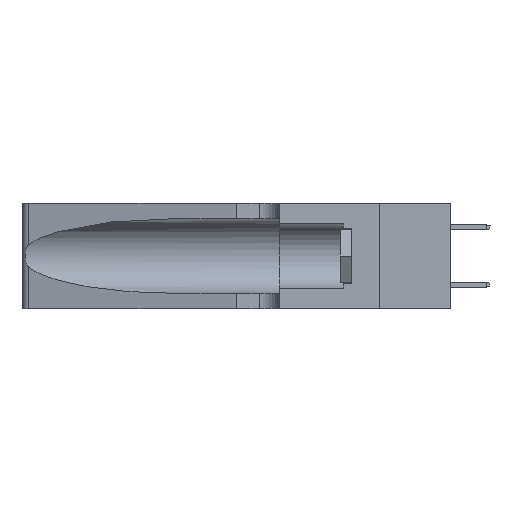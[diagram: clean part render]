
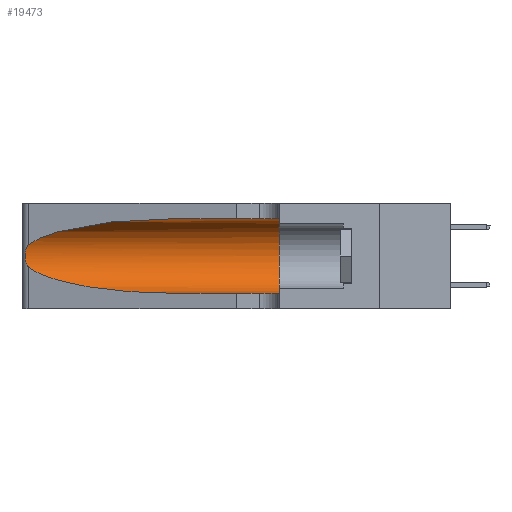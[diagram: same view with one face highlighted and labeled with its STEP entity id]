
A CAD part, left-side view. The second image highlights one B-rep face of the part: STEP entity #19473.
In plain terms, the highlighted cylindrical face has radius 3.308 mm (diameter 6.617 mm), a partial arc.
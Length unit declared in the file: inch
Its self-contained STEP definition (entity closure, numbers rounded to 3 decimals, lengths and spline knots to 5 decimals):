
#11 = EDGE_CURVE ( 'NONE', #1694, #17740, #10269, .T. ) ;
#642 = AXIS2_PLACEMENT_3D ( 'NONE', #17769, #10999, #1192 ) ;
#1048 = AXIS2_PLACEMENT_3D ( 'NONE', #8635, #15375, #2091 ) ;
#1192 = DIRECTION ( 'NONE',  ( 0., 0., 1. ) ) ;
#1694 = VERTEX_POINT ( 'NONE', #3287 ) ;
#1867 = CARTESIAN_POINT ( 'NONE',  ( 0.25487, 1.22718, 0.22369 ) ) ;
#2091 = DIRECTION ( 'NONE',  ( 0., 0., -1. ) ) ;
#2118 = ORIENTED_EDGE ( 'NONE', *, *, #17511, .F. ) ;
#2253 = CARTESIAN_POINT ( 'NONE',  ( 0.26018, 1.23835, 0.19895 ) ) ;
#2735 = ORIENTED_EDGE ( 'NONE', *, *, #10986, .T. ) ;
#3287 = CARTESIAN_POINT ( 'NONE',  ( 0.1305, 0.72297, 0.31525 ) ) ;
#4034 = VERTEX_POINT ( 'NONE', #18263 ) ;
#4070 = EDGE_CURVE ( 'NONE', #19789, #4034, #12490, .T. ) ;
#4554 = CARTESIAN_POINT ( 'NONE',  ( 0.25487, 1.22718, 0.22369 ) ) ;
#4856 = EDGE_CURVE ( 'NONE', #4034, #5513, #12117, .T. ) ;
#4936 = VECTOR ( 'NONE', #10066, 39.37008 ) ;
#5051 = CARTESIAN_POINT ( 'NONE',  ( 0.18966, 0.96281, 0.05475 ) ) ;
#5262 = B_SPLINE_CURVE_WITH_KNOTS ( 'NONE', 3,
 ( #8900, #7268, #17388, #8787, #19178, #2253, #9233, #17286, #14027, #12148, #9009, #14141, #15643, #20813 ),
 .UNSPECIFIED., .F., .F.,
 ( 4, 2, 2, 2, 2, 2, 4 ),
 ( 0., 0.00027, 0.00053, 0.00107, 0.0016, 0.00187, 0.00214 ),
 .UNSPECIFIED. ) ;
#5513 = VERTEX_POINT ( 'NONE', #20070 ) ;
#6679 = CARTESIAN_POINT ( 'NONE',  ( 0.25487, 1.22718, 0.14631 ) ) ;
#7016 = CARTESIAN_POINT ( 'NONE',  ( 0.1305, 1.61858, 0.05475 ) ) ;
#7235 = CARTESIAN_POINT ( 'NONE',  ( 0.1305, 0.72297, 0.05475 ) ) ;
#7268 = CARTESIAN_POINT ( 'NONE',  ( 0.25555, 1.22994, 0.2215 ) ) ;
#7604 = CIRCLE ( 'NONE', #642, 0.13025 ) ;
#8635 = CARTESIAN_POINT ( 'NONE',  ( 0.1305, 1.61858, 0.185 ) ) ;
#8733 = CARTESIAN_POINT ( 'NONE',  ( 0.18966, 0.96281, 0.31525 ) ) ;
#8787 = CARTESIAN_POINT ( 'NONE',  ( 0.25787, 1.23484, 0.2124 ) ) ;
#8900 = CARTESIAN_POINT ( 'NONE',  ( 0.25487, 1.22718, 0.22369 ) ) ;
#9009 = CARTESIAN_POINT ( 'NONE',  ( 0.25789, 1.23486, 0.15765 ) ) ;
#9233 = CARTESIAN_POINT ( 'NONE',  ( 0.26075, 1.23896, 0.19203 ) ) ;
#10039 = CARTESIAN_POINT ( 'NONE',  ( 0.1305, 0.72297, 0.31525 ) ) ;
#10066 = DIRECTION ( 'NONE',  ( 0., -1., 0. ) ) ;
#10269 =( BOUNDED_CURVE ( )  B_SPLINE_CURVE ( 3, ( #10039, #8733, #13522, #1867 ),
 .UNSPECIFIED., .F., .T. ) 
 B_SPLINE_CURVE_WITH_KNOTS ( ( 4, 4 ),
 ( 1.5708, 2.84003 ),
 .UNSPECIFIED. ) 
 CURVE ( )  GEOMETRIC_REPRESENTATION_ITEM ( )  RATIONAL_B_SPLINE_CURVE ( ( 1., 0.87, 0.87, 1. ) ) 
 REPRESENTATION_ITEM ( '' )  );
#10433 = LINE ( 'NONE', #10548, #14216 ) ;
#10465 = VERTEX_POINT ( 'NONE', #18112 ) ;
#10548 = CARTESIAN_POINT ( 'NONE',  ( 0.1305, 1.61858, 0.31525 ) ) ;
#10735 = EDGE_LOOP ( 'NONE', ( #14231, #2735, #16268, #14659, #14898, #2118 ) ) ;
#10986 = EDGE_CURVE ( 'NONE', #17740, #19789, #5262, .T. ) ;
#10999 = DIRECTION ( 'NONE',  ( 0., 1., 0. ) ) ;
#11883 = FACE_OUTER_BOUND ( 'NONE', #10735, .T. ) ;
#12117 = LINE ( 'NONE', #7016, #4936 ) ;
#12148 = CARTESIAN_POINT ( 'NONE',  ( 0.25856, 1.23593, 0.16098 ) ) ;
#12490 =( BOUNDED_CURVE ( )  B_SPLINE_CURVE ( 3, ( #6679, #13332, #5051, #7235 ),
 .UNSPECIFIED., .F., .T. ) 
 B_SPLINE_CURVE_WITH_KNOTS ( ( 4, 4 ),
 ( 3.44316, 4.71239 ),
 .UNSPECIFIED. ) 
 CURVE ( )  GEOMETRIC_REPRESENTATION_ITEM ( )  RATIONAL_B_SPLINE_CURVE ( ( 1., 0.87, 0.87, 1. ) ) 
 REPRESENTATION_ITEM ( '' )  );
#13332 = CARTESIAN_POINT ( 'NONE',  ( 0.2373, 1.15595, 0.08982 ) ) ;
#13522 = CARTESIAN_POINT ( 'NONE',  ( 0.2373, 1.15595, 0.28018 ) ) ;
#14027 = CARTESIAN_POINT ( 'NONE',  ( 0.26017, 1.23833, 0.17102 ) ) ;
#14141 = CARTESIAN_POINT ( 'NONE',  ( 0.25639, 1.23186, 0.15144 ) ) ;
#14216 = VECTOR ( 'NONE', #18528, 39.37008 ) ;
#14231 = ORIENTED_EDGE ( 'NONE', *, *, #11, .T. ) ;
#14659 = ORIENTED_EDGE ( 'NONE', *, *, #4856, .T. ) ;
#14898 = ORIENTED_EDGE ( 'NONE', *, *, #17241, .F. ) ;
#15375 = DIRECTION ( 'NONE',  ( 0., -1., 0. ) ) ;
#15643 = CARTESIAN_POINT ( 'NONE',  ( 0.25555, 1.22993, 0.14849 ) ) ;
#16268 = ORIENTED_EDGE ( 'NONE', *, *, #4070, .T. ) ;
#17241 = EDGE_CURVE ( 'NONE', #10465, #5513, #7604, .T. ) ;
#17286 = CARTESIAN_POINT ( 'NONE',  ( 0.26075, 1.23896, 0.178 ) ) ;
#17388 = CARTESIAN_POINT ( 'NONE',  ( 0.25639, 1.23184, 0.21858 ) ) ;
#17511 = EDGE_CURVE ( 'NONE', #1694, #10465, #10433, .T. ) ;
#17740 = VERTEX_POINT ( 'NONE', #4554 ) ;
#17769 = CARTESIAN_POINT ( 'NONE',  ( 0.1305, 0.35, 0.185 ) ) ;
#18112 = CARTESIAN_POINT ( 'NONE',  ( 0.1305, 0.35, 0.31525 ) ) ;
#18263 = CARTESIAN_POINT ( 'NONE',  ( 0.1305, 0.72297, 0.05475 ) ) ;
#18465 = CYLINDRICAL_SURFACE ( 'NONE', #1048, 0.13025 ) ;
#18528 = DIRECTION ( 'NONE',  ( 0., -1., 0. ) ) ;
#19178 = CARTESIAN_POINT ( 'NONE',  ( 0.25854, 1.2359, 0.20912 ) ) ;
#19473 = ADVANCED_FACE ( 'NONE', ( #11883 ), #18465, .F. ) ;
#19789 = VERTEX_POINT ( 'NONE', #20744 ) ;
#20070 = CARTESIAN_POINT ( 'NONE',  ( 0.1305, 0.35, 0.05475 ) ) ;
#20744 = CARTESIAN_POINT ( 'NONE',  ( 0.25487, 1.22718, 0.14631 ) ) ;
#20813 = CARTESIAN_POINT ( 'NONE',  ( 0.25487, 1.22718, 0.14631 ) ) ;
